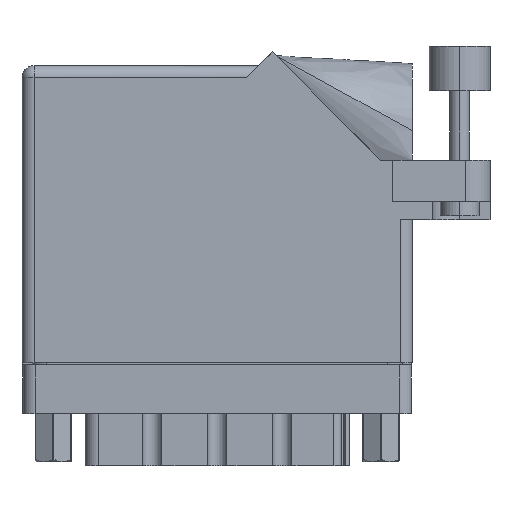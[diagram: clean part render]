
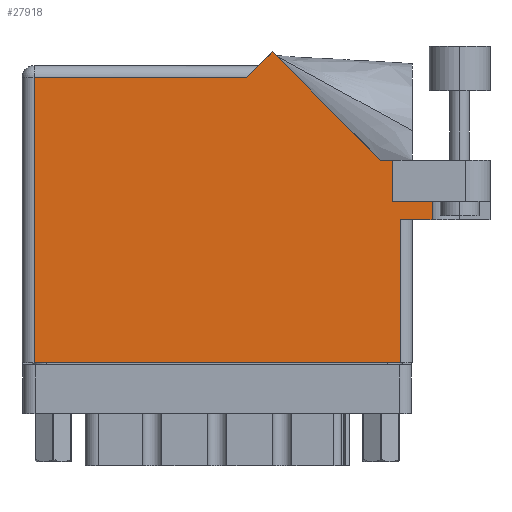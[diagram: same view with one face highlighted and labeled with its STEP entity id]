
A CAD part, front view. The second image highlights one B-rep face of the part: STEP entity #27918.
In plain terms, the highlighted face is planar.
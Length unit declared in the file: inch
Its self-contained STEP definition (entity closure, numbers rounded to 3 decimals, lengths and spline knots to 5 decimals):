
#835 = DIRECTION ( 'NONE',  ( 0., 1., 0. ) ) ;
#1135 = FACE_OUTER_BOUND ( 'NONE', #34369, .T. ) ;
#1388 = LINE ( 'NONE', #14476, #15910 ) ;
#1682 = CARTESIAN_POINT ( 'NONE',  ( 0., 1.53, 0. ) ) ;
#2213 = VERTEX_POINT ( 'NONE', #25377 ) ;
#2965 = DIRECTION ( 'NONE',  ( -1., 0., 0. ) ) ;
#3018 = VERTEX_POINT ( 'NONE', #30750 ) ;
#3148 = EDGE_CURVE ( 'NONE', #11578, #2213, #17090, .T. ) ;
#3721 = VERTEX_POINT ( 'NONE', #30497 ) ;
#4160 = DIRECTION ( 'NONE',  ( 1., 0., 0. ) ) ;
#5591 = VERTEX_POINT ( 'NONE', #31927 ) ;
#7050 = ORIENTED_EDGE ( 'NONE', *, *, #35105, .T. ) ;
#7702 = ORIENTED_EDGE ( 'NONE', *, *, #45742, .T. ) ;
#7732 = DIRECTION ( 'NONE',  ( 0., -1., 0. ) ) ;
#8230 = LINE ( 'NONE', #24767, #26415 ) ;
#8394 = ORIENTED_EDGE ( 'NONE', *, *, #15202, .T. ) ;
#9829 = LINE ( 'NONE', #28083, #18902 ) ;
#9868 = VERTEX_POINT ( 'NONE', #10669 ) ;
#10669 = CARTESIAN_POINT ( 'NONE',  ( 1.948, 0.737, 0. ) ) ;
#11578 = VERTEX_POINT ( 'NONE', #37480 ) ;
#11834 = VECTOR ( 'NONE', #31918, 39.37008 ) ;
#11867 = DIRECTION ( 'NONE',  ( 1., 0., 0. ) ) ;
#12283 = CARTESIAN_POINT ( 'NONE',  ( 2.01, 0.737, 0. ) ) ;
#12327 = EDGE_CURVE ( 'NONE', #27011, #3018, #19339, .T. ) ;
#13019 = DIRECTION ( 'NONE',  ( 0., 0., -1. ) ) ;
#13043 = EDGE_CURVE ( 'NONE', #48014, #22340, #19809, .T. ) ;
#13129 = CARTESIAN_POINT ( 'NONE',  ( 2.1115, 1.16177, 0. ) ) ;
#14476 = CARTESIAN_POINT ( 'NONE',  ( 0., 1.468, 0. ) ) ;
#14624 = CARTESIAN_POINT ( 'NONE',  ( 1.155, 1.468, 0. ) ) ;
#15136 = CARTESIAN_POINT ( 'NONE',  ( 1.948, 0., 0. ) ) ;
#15202 = EDGE_CURVE ( 'NONE', #3721, #27011, #8230, .T. ) ;
#15741 = CARTESIAN_POINT ( 'NONE',  ( 1.91, 0.831, 0. ) ) ;
#15910 = VECTOR ( 'NONE', #2965, 39.37008 ) ;
#16118 = LINE ( 'NONE', #26391, #39170 ) ;
#17090 = LINE ( 'NONE', #13129, #34077 ) ;
#17889 = LINE ( 'NONE', #12283, #11834 ) ;
#18604 = VECTOR ( 'NONE', #4160, 39.37008 ) ;
#18902 = VECTOR ( 'NONE', #835, 39.37008 ) ;
#19050 = CARTESIAN_POINT ( 'NONE',  ( 0.062, 0., 0. ) ) ;
#19183 = ORIENTED_EDGE ( 'NONE', *, *, #21498, .T. ) ;
#19339 = LINE ( 'NONE', #43020, #42931 ) ;
#19809 = LINE ( 'NONE', #31277, #18604 ) ;
#20600 = EDGE_CURVE ( 'NONE', #22340, #9868, #34787, .T. ) ;
#20776 = DIRECTION ( 'NONE',  ( 0., 1., 0. ) ) ;
#21498 = EDGE_CURVE ( 'NONE', #33247, #5591, #1388, .T. ) ;
#22340 = VERTEX_POINT ( 'NONE', #15136 ) ;
#22415 = ORIENTED_EDGE ( 'NONE', *, *, #46698, .F. ) ;
#23860 = CARTESIAN_POINT ( 'NONE',  ( 1.91, 0.831, 0. ) ) ;
#24767 = CARTESIAN_POINT ( 'NONE',  ( 2.41, 1.044, 0. ) ) ;
#25377 = CARTESIAN_POINT ( 'NONE',  ( 2.1115, 0.737, 0. ) ) ;
#26391 = CARTESIAN_POINT ( 'NONE',  ( 1.217, 1.53, 0. ) ) ;
#26415 = VECTOR ( 'NONE', #32916, 39.37008 ) ;
#27011 = VERTEX_POINT ( 'NONE', #44275 ) ;
#27199 = ORIENTED_EDGE ( 'NONE', *, *, #3148, .F. ) ;
#27460 = AXIS2_PLACEMENT_3D ( 'NONE', #1682, #13019, #40109 ) ;
#27918 = ADVANCED_FACE ( 'NONE', ( #1135 ), #39956, .F. ) ;
#28083 = CARTESIAN_POINT ( 'NONE',  ( 1.91, 0.831, 0. ) ) ;
#30497 = CARTESIAN_POINT ( 'NONE',  ( 1.91, 1.044, 0. ) ) ;
#30579 = VECTOR ( 'NONE', #20776, 39.37008 ) ;
#30750 = CARTESIAN_POINT ( 'NONE',  ( 1.28771, 1.60071, 0. ) ) ;
#30952 = CARTESIAN_POINT ( 'NONE',  ( 0.062, 0., 0. ) ) ;
#31155 = DIRECTION ( 'NONE',  ( -0.707, 0.707, 0. ) ) ;
#31277 = CARTESIAN_POINT ( 'NONE',  ( 0., 0., 0. ) ) ;
#31918 = DIRECTION ( 'NONE',  ( 1., 0., 0. ) ) ;
#31927 = CARTESIAN_POINT ( 'NONE',  ( 0.062, 1.468, 0. ) ) ;
#32916 = DIRECTION ( 'NONE',  ( -1., 0., 0. ) ) ;
#33247 = VERTEX_POINT ( 'NONE', #14624 ) ;
#33829 = ORIENTED_EDGE ( 'NONE', *, *, #47522, .T. ) ;
#34035 = DIRECTION ( 'NONE',  ( -0.707, -0.707, 0. ) ) ;
#34077 = VECTOR ( 'NONE', #40216, 39.37008 ) ;
#34369 = EDGE_LOOP ( 'NONE', ( #48996, #45170, #33829, #27199, #22415, #7050, #8394, #41700, #7702, #19183, #46906 ) ) ;
#34787 = LINE ( 'NONE', #43381, #30579 ) ;
#35105 = EDGE_CURVE ( 'NONE', #50197, #3721, #9829, .T. ) ;
#37480 = CARTESIAN_POINT ( 'NONE',  ( 2.1115, 0.831, 0. ) ) ;
#39170 = VECTOR ( 'NONE', #34035, 39.37008 ) ;
#39956 = PLANE ( 'NONE',  #27460 ) ;
#40109 = DIRECTION ( 'NONE',  ( -1., 0., 0. ) ) ;
#40216 = DIRECTION ( 'NONE',  ( 0., -1., 0. ) ) ;
#41472 = EDGE_CURVE ( 'NONE', #5591, #48014, #42526, .T. ) ;
#41700 = ORIENTED_EDGE ( 'NONE', *, *, #12327, .T. ) ;
#42526 = LINE ( 'NONE', #30952, #44914 ) ;
#42931 = VECTOR ( 'NONE', #31155, 39.37008 ) ;
#43020 = CARTESIAN_POINT ( 'NONE',  ( 1.84442, 1.044, 0. ) ) ;
#43381 = CARTESIAN_POINT ( 'NONE',  ( 1.948, 0.737, 0. ) ) ;
#44275 = CARTESIAN_POINT ( 'NONE',  ( 1.84442, 1.044, 0. ) ) ;
#44914 = VECTOR ( 'NONE', #7732, 39.37008 ) ;
#45170 = ORIENTED_EDGE ( 'NONE', *, *, #20600, .T. ) ;
#45742 = EDGE_CURVE ( 'NONE', #3018, #33247, #16118, .T. ) ;
#46383 = VECTOR ( 'NONE', #11867, 39.37008 ) ;
#46698 = EDGE_CURVE ( 'NONE', #50197, #11578, #49399, .T. ) ;
#46906 = ORIENTED_EDGE ( 'NONE', *, *, #41472, .T. ) ;
#47522 = EDGE_CURVE ( 'NONE', #9868, #2213, #17889, .T. ) ;
#48014 = VERTEX_POINT ( 'NONE', #19050 ) ;
#48996 = ORIENTED_EDGE ( 'NONE', *, *, #13043, .T. ) ;
#49399 = LINE ( 'NONE', #15741, #46383 ) ;
#50197 = VERTEX_POINT ( 'NONE', #23860 ) ;
